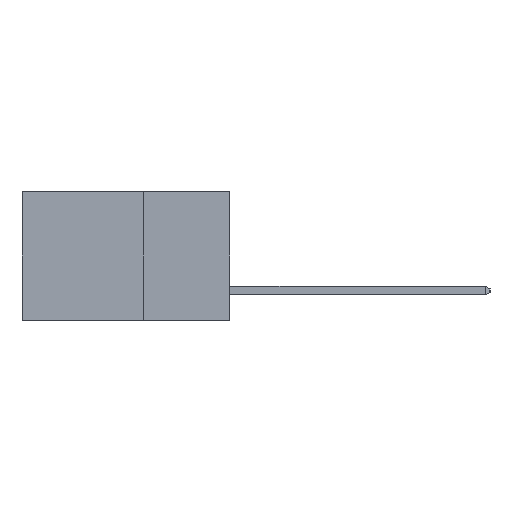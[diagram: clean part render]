
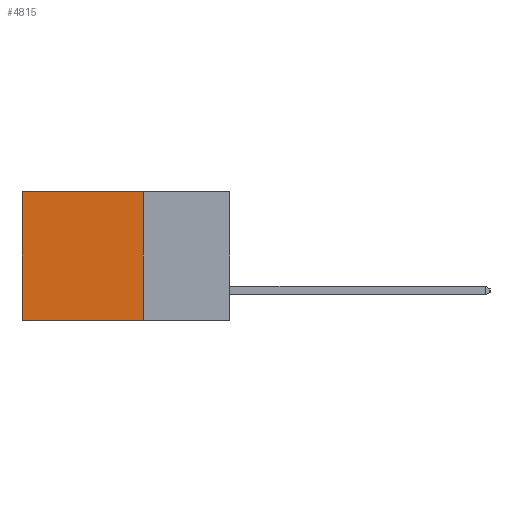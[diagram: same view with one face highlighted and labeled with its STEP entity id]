
A CAD part, left-side view. The second image highlights one B-rep face of the part: STEP entity #4815.
In plain terms, the highlighted planar face has unit normal (-1, 0, 0).
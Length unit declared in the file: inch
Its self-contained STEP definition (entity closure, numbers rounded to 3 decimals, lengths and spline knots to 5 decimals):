
#58 = EDGE_LOOP ( 'NONE', ( #11819, #11587, #7978, #11550 ) ) ;
#258 = VERTEX_POINT ( 'NONE', #11638 ) ;
#674 = VERTEX_POINT ( 'NONE', #7039 ) ;
#715 = DIRECTION ( 'NONE',  ( 1., 0., 0. ) ) ;
#1020 = DIRECTION ( 'NONE',  ( 0., 0., -1. ) ) ;
#1108 = PLANE ( 'NONE',  #11775 ) ;
#2076 = FACE_OUTER_BOUND ( 'NONE', #58, .T. ) ;
#2077 = CARTESIAN_POINT ( 'NONE',  ( 0.298, 0.6, 0. ) ) ;
#3686 = CARTESIAN_POINT ( 'NONE',  ( 0.298, 0.25, -0.37 ) ) ;
#3698 = DIRECTION ( 'NONE',  ( 0., 0., -1. ) ) ;
#3734 = VECTOR ( 'NONE', #8074, 39.37008 ) ;
#3930 = CARTESIAN_POINT ( 'NONE',  ( 0.298, 0.6, 0. ) ) ;
#4432 = EDGE_CURVE ( 'NONE', #674, #8958, #6491, .T. ) ;
#4745 = VECTOR ( 'NONE', #3698, 39.37008 ) ;
#4815 = ADVANCED_FACE ( 'NONE', ( #2076 ), #1108, .F. ) ;
#5730 = VERTEX_POINT ( 'NONE', #3686 ) ;
#6491 = LINE ( 'NONE', #7938, #3734 ) ;
#6608 = VECTOR ( 'NONE', #7703, 39.37008 ) ;
#7039 = CARTESIAN_POINT ( 'NONE',  ( 0.298, 0.25, 0. ) ) ;
#7703 = DIRECTION ( 'NONE',  ( 0., 1., 0. ) ) ;
#7744 = CARTESIAN_POINT ( 'NONE',  ( 0.298, 0.25, -0.37 ) ) ;
#7938 = CARTESIAN_POINT ( 'NONE',  ( 0.298, 0.25, 0. ) ) ;
#7978 = ORIENTED_EDGE ( 'NONE', *, *, #8725, .F. ) ;
#8074 = DIRECTION ( 'NONE',  ( 0., 1., 0. ) ) ;
#8268 = EDGE_CURVE ( 'NONE', #5730, #258, #9010, .T. ) ;
#8696 = VECTOR ( 'NONE', #9441, 39.37008 ) ;
#8725 = EDGE_CURVE ( 'NONE', #674, #5730, #11828, .T. ) ;
#8958 = VERTEX_POINT ( 'NONE', #3930 ) ;
#9010 = LINE ( 'NONE', #7744, #6608 ) ;
#9162 = CARTESIAN_POINT ( 'NONE',  ( 0.298, 0.25, 0. ) ) ;
#9441 = DIRECTION ( 'NONE',  ( 0., 0., -1. ) ) ;
#10513 = EDGE_CURVE ( 'NONE', #8958, #258, #11296, .T. ) ;
#11296 = LINE ( 'NONE', #2077, #8696 ) ;
#11441 = CARTESIAN_POINT ( 'NONE',  ( 0.298, 0.25, 0. ) ) ;
#11550 = ORIENTED_EDGE ( 'NONE', *, *, #4432, .T. ) ;
#11587 = ORIENTED_EDGE ( 'NONE', *, *, #8268, .F. ) ;
#11638 = CARTESIAN_POINT ( 'NONE',  ( 0.298, 0.6, -0.37 ) ) ;
#11775 = AXIS2_PLACEMENT_3D ( 'NONE', #11441, #715, #1020 ) ;
#11819 = ORIENTED_EDGE ( 'NONE', *, *, #10513, .T. ) ;
#11828 = LINE ( 'NONE', #9162, #4745 ) ;
